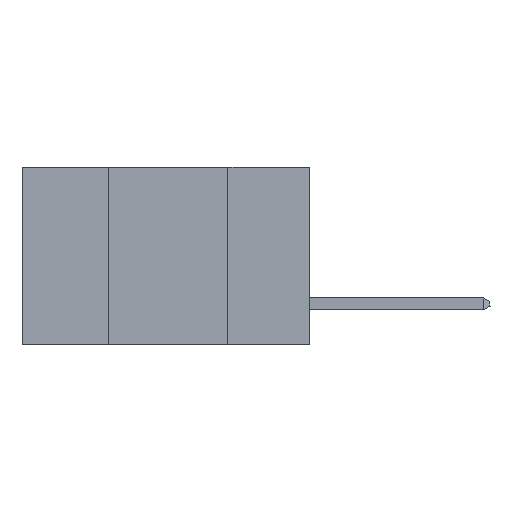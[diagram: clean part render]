
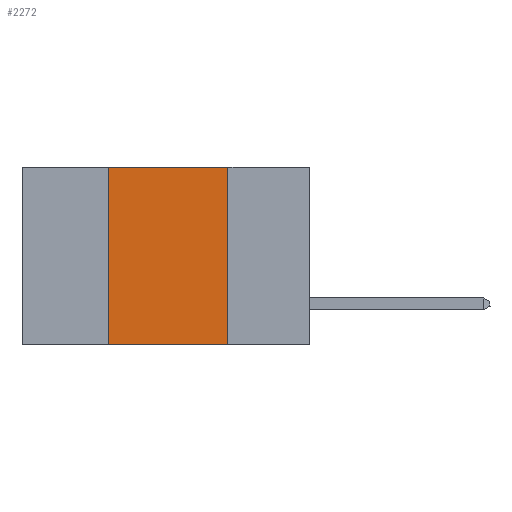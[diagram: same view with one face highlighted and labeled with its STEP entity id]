
A CAD part, left-side view. The second image highlights one B-rep face of the part: STEP entity #2272.
In plain terms, the highlighted planar face has unit normal (-1, 0, 0).
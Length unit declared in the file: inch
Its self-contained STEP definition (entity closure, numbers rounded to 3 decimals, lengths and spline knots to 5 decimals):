
#67 = EDGE_CURVE ( 'NONE', #22385, #931, #4675, .T. ) ;
#931 = VERTEX_POINT ( 'NONE', #13961 ) ;
#2272 = ADVANCED_FACE ( 'NONE', ( #22498 ), #17482, .F. ) ;
#2635 = VECTOR ( 'NONE', #4150, 39.37008 ) ;
#3579 = ORIENTED_EDGE ( 'NONE', *, *, #23916, .F. ) ;
#3985 = ORIENTED_EDGE ( 'NONE', *, *, #15531, .T. ) ;
#4090 = CARTESIAN_POINT ( 'NONE',  ( 0., 0.17, 0. ) ) ;
#4150 = DIRECTION ( 'NONE',  ( 0., -1., 0. ) ) ;
#4675 = LINE ( 'NONE', #4090, #8409 ) ;
#4919 = DIRECTION ( 'NONE',  ( 0., -1., 0. ) ) ;
#5681 = DIRECTION ( 'NONE',  ( 0., 0., -1. ) ) ;
#6151 = LINE ( 'NONE', #6471, #16252 ) ;
#6389 = EDGE_LOOP ( 'NONE', ( #12622, #11907, #3579, #3985 ) ) ;
#6471 = CARTESIAN_POINT ( 'NONE',  ( 0., 0.42, 0. ) ) ;
#6879 = VECTOR ( 'NONE', #4919, 39.37008 ) ;
#7554 = LINE ( 'NONE', #13534, #6879 ) ;
#8409 = VECTOR ( 'NONE', #12436, 39.37008 ) ;
#8417 = CARTESIAN_POINT ( 'NONE',  ( 0., 0.6, 0. ) ) ;
#8519 = VERTEX_POINT ( 'NONE', #26193 ) ;
#8789 = CARTESIAN_POINT ( 'NONE',  ( 0., 0.6, 0. ) ) ;
#11907 = ORIENTED_EDGE ( 'NONE', *, *, #24993, .F. ) ;
#12436 = DIRECTION ( 'NONE',  ( 0., 0., -1. ) ) ;
#12622 = ORIENTED_EDGE ( 'NONE', *, *, #67, .F. ) ;
#12910 = VERTEX_POINT ( 'NONE', #23674 ) ;
#13534 = CARTESIAN_POINT ( 'NONE',  ( 0., 0.6, -0.37 ) ) ;
#13961 = CARTESIAN_POINT ( 'NONE',  ( 0., 0.17, -0.37 ) ) ;
#15205 = LINE ( 'NONE', #8789, #2635 ) ;
#15531 = EDGE_CURVE ( 'NONE', #8519, #931, #7554, .T. ) ;
#16252 = VECTOR ( 'NONE', #21547, 39.37008 ) ;
#17482 = PLANE ( 'NONE',  #18875 ) ;
#18875 = AXIS2_PLACEMENT_3D ( 'NONE', #8417, #27923, #5681 ) ;
#19121 = CARTESIAN_POINT ( 'NONE',  ( 0., 0.17, 0. ) ) ;
#21547 = DIRECTION ( 'NONE',  ( 0., 0., 1. ) ) ;
#22385 = VERTEX_POINT ( 'NONE', #19121 ) ;
#22498 = FACE_OUTER_BOUND ( 'NONE', #6389, .T. ) ;
#23674 = CARTESIAN_POINT ( 'NONE',  ( 0., 0.42, 0. ) ) ;
#23916 = EDGE_CURVE ( 'NONE', #8519, #12910, #6151, .T. ) ;
#24993 = EDGE_CURVE ( 'NONE', #12910, #22385, #15205, .T. ) ;
#26193 = CARTESIAN_POINT ( 'NONE',  ( 0., 0.42, -0.37 ) ) ;
#27923 = DIRECTION ( 'NONE',  ( 1., 0., 0. ) ) ;
